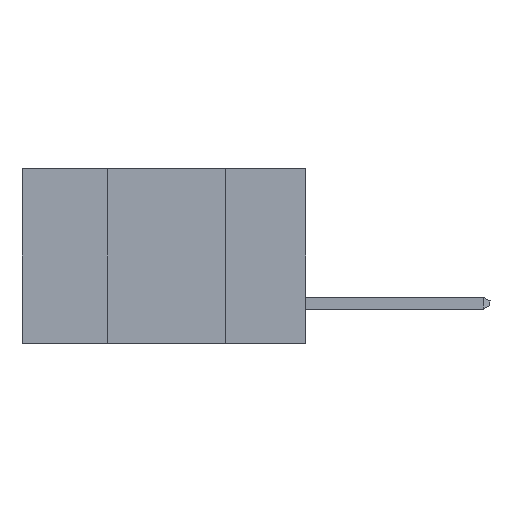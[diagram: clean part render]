
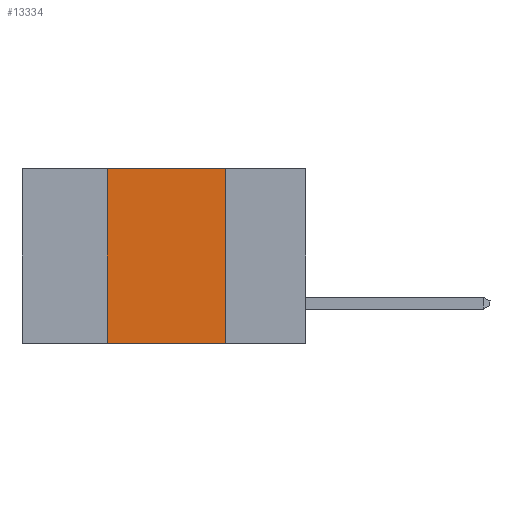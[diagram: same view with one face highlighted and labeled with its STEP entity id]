
A CAD part, left-side view. The second image highlights one B-rep face of the part: STEP entity #13334.
In plain terms, the highlighted planar face has unit normal (-1, 0, 0).
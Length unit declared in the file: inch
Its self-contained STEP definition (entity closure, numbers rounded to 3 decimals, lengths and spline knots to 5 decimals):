
#1363 = CARTESIAN_POINT ( 'NONE',  ( 0., 0.6, 0. ) ) ;
#1423 = CARTESIAN_POINT ( 'NONE',  ( 0., 0.42, -0.37 ) ) ;
#1694 = CARTESIAN_POINT ( 'NONE',  ( 0., 0.42, -0.37 ) ) ;
#3395 = PLANE ( 'NONE',  #19075 ) ;
#3544 = DIRECTION ( 'NONE',  ( 0., 0., 1. ) ) ;
#4880 = FACE_OUTER_BOUND ( 'NONE', #11978, .T. ) ;
#5267 = VERTEX_POINT ( 'NONE', #20012 ) ;
#6115 = ORIENTED_EDGE ( 'NONE', *, *, #9857, .F. ) ;
#6234 = ORIENTED_EDGE ( 'NONE', *, *, #14192, .F. ) ;
#6867 = VECTOR ( 'NONE', #14302, 39.37008 ) ;
#7261 = DIRECTION ( 'NONE',  ( 0., 0., -1. ) ) ;
#9857 = EDGE_CURVE ( 'NONE', #17470, #12144, #16619, .T. ) ;
#10375 = VECTOR ( 'NONE', #7261, 39.37008 ) ;
#10560 = CARTESIAN_POINT ( 'NONE',  ( 0., 0.6, -0.37 ) ) ;
#11117 = EDGE_CURVE ( 'NONE', #16027, #12144, #15851, .T. ) ;
#11978 = EDGE_LOOP ( 'NONE', ( #6115, #6234, #13101, #16053 ) ) ;
#12118 = EDGE_CURVE ( 'NONE', #16027, #5267, #22196, .T. ) ;
#12144 = VERTEX_POINT ( 'NONE', #22451 ) ;
#12405 = CARTESIAN_POINT ( 'NONE',  ( 0., 0.6, 0. ) ) ;
#12673 = CARTESIAN_POINT ( 'NONE',  ( 0., 0.17, -0.37 ) ) ;
#13101 = ORIENTED_EDGE ( 'NONE', *, *, #12118, .F. ) ;
#13334 = ADVANCED_FACE ( 'NONE', ( #4880 ), #3395, .F. ) ;
#13480 = VECTOR ( 'NONE', #3544, 39.37008 ) ;
#14126 = DIRECTION ( 'NONE',  ( 1., 0., 0. ) ) ;
#14192 = EDGE_CURVE ( 'NONE', #5267, #17470, #16159, .T. ) ;
#14302 = DIRECTION ( 'NONE',  ( 0., -1., 0. ) ) ;
#15851 = LINE ( 'NONE', #10560, #23350 ) ;
#16027 = VERTEX_POINT ( 'NONE', #1423 ) ;
#16053 = ORIENTED_EDGE ( 'NONE', *, *, #11117, .T. ) ;
#16159 = LINE ( 'NONE', #1363, #6867 ) ;
#16619 = LINE ( 'NONE', #12673, #10375 ) ;
#17470 = VERTEX_POINT ( 'NONE', #20946 ) ;
#17589 = DIRECTION ( 'NONE',  ( 0., -1., 0. ) ) ;
#19075 = AXIS2_PLACEMENT_3D ( 'NONE', #12405, #14126, #19938 ) ;
#19938 = DIRECTION ( 'NONE',  ( 0., 0., -1. ) ) ;
#20012 = CARTESIAN_POINT ( 'NONE',  ( 0., 0.42, 0. ) ) ;
#20946 = CARTESIAN_POINT ( 'NONE',  ( 0., 0.17, 0. ) ) ;
#22196 = LINE ( 'NONE', #1694, #13480 ) ;
#22451 = CARTESIAN_POINT ( 'NONE',  ( 0., 0.17, -0.37 ) ) ;
#23350 = VECTOR ( 'NONE', #17589, 39.37008 ) ;
